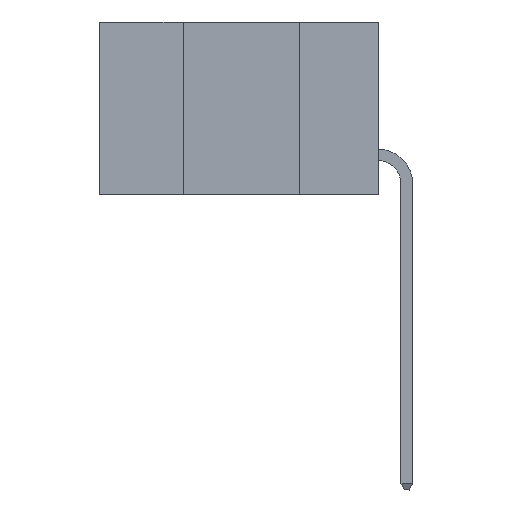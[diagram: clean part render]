
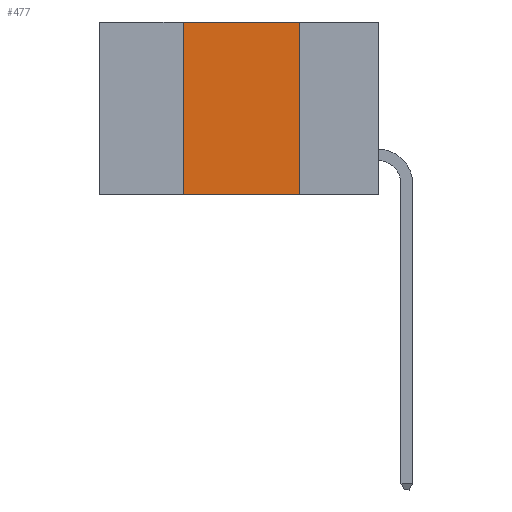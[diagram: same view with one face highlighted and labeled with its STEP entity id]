
A CAD part, left-side view. The second image highlights one B-rep face of the part: STEP entity #477.
In plain terms, the highlighted planar face has unit normal (-1, 0, 0).
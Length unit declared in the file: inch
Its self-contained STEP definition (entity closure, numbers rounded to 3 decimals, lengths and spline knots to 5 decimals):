
#12 = CARTESIAN_POINT ( 'NONE',  ( 0., 0.6, -0.37 ) ) ;
#35 = DIRECTION ( 'NONE',  ( 1., 0., 0. ) ) ;
#37 = VERTEX_POINT ( 'NONE', #7414 ) ;
#100 = EDGE_CURVE ( 'NONE', #1322, #10618, #2716, .T. ) ;
#319 = EDGE_LOOP ( 'NONE', ( #7765, #4553, #7709, #1955 ) ) ;
#474 = VECTOR ( 'NONE', #2391, 39.37008 ) ;
#477 = ADVANCED_FACE ( 'NONE', ( #7743 ), #1741, .F. ) ;
#796 = EDGE_CURVE ( 'NONE', #1243, #37, #1497, .T. ) ;
#1010 = VECTOR ( 'NONE', #6243, 39.37008 ) ;
#1243 = VERTEX_POINT ( 'NONE', #6916 ) ;
#1322 = VERTEX_POINT ( 'NONE', #9466 ) ;
#1497 = LINE ( 'NONE', #7439, #474 ) ;
#1741 = PLANE ( 'NONE',  #4330 ) ;
#1955 = ORIENTED_EDGE ( 'NONE', *, *, #4048, .T. ) ;
#2391 = DIRECTION ( 'NONE',  ( 0., 0., 1. ) ) ;
#2716 = LINE ( 'NONE', #4489, #1010 ) ;
#4048 = EDGE_CURVE ( 'NONE', #1243, #10618, #6091, .T. ) ;
#4327 = DIRECTION ( 'NONE',  ( 0., -1., 0. ) ) ;
#4330 = AXIS2_PLACEMENT_3D ( 'NONE', #4460, #35, #6899 ) ;
#4460 = CARTESIAN_POINT ( 'NONE',  ( 0., 0.6, 0. ) ) ;
#4489 = CARTESIAN_POINT ( 'NONE',  ( 0., 0.17, -0.37 ) ) ;
#4553 = ORIENTED_EDGE ( 'NONE', *, *, #9594, .F. ) ;
#5554 = VECTOR ( 'NONE', #8745, 39.37008 ) ;
#5603 = CARTESIAN_POINT ( 'NONE',  ( 0., 0.17, -0.37 ) ) ;
#6091 = LINE ( 'NONE', #12, #5554 ) ;
#6190 = CARTESIAN_POINT ( 'NONE',  ( 0., 0.6, 0. ) ) ;
#6243 = DIRECTION ( 'NONE',  ( 0., 0., -1. ) ) ;
#6899 = DIRECTION ( 'NONE',  ( 0., 0., -1. ) ) ;
#6916 = CARTESIAN_POINT ( 'NONE',  ( 0., 0.42, -0.37 ) ) ;
#7414 = CARTESIAN_POINT ( 'NONE',  ( 0., 0.42, 0. ) ) ;
#7439 = CARTESIAN_POINT ( 'NONE',  ( 0., 0.42, -0.37 ) ) ;
#7709 = ORIENTED_EDGE ( 'NONE', *, *, #796, .F. ) ;
#7743 = FACE_OUTER_BOUND ( 'NONE', #319, .T. ) ;
#7765 = ORIENTED_EDGE ( 'NONE', *, *, #100, .F. ) ;
#8022 = VECTOR ( 'NONE', #4327, 39.37008 ) ;
#8745 = DIRECTION ( 'NONE',  ( 0., -1., 0. ) ) ;
#9426 = LINE ( 'NONE', #6190, #8022 ) ;
#9466 = CARTESIAN_POINT ( 'NONE',  ( 0., 0.17, 0. ) ) ;
#9594 = EDGE_CURVE ( 'NONE', #37, #1322, #9426, .T. ) ;
#10618 = VERTEX_POINT ( 'NONE', #5603 ) ;
